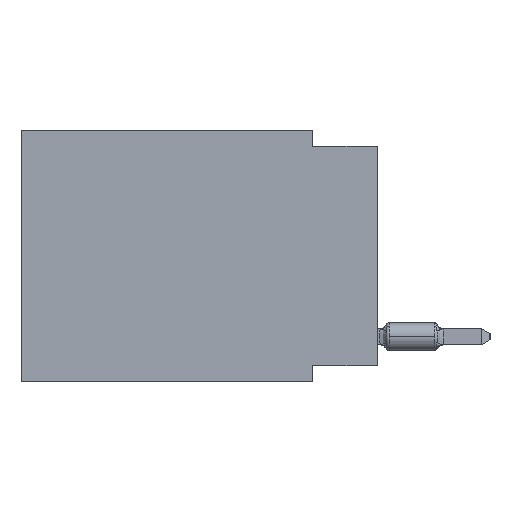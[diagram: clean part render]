
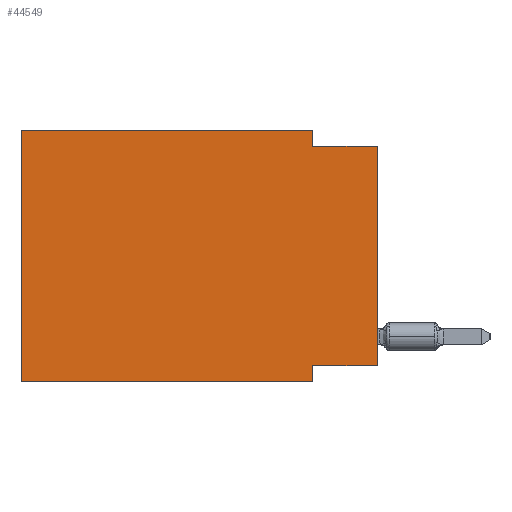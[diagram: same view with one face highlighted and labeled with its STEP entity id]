
A CAD part, left-side view. The second image highlights one B-rep face of the part: STEP entity #44549.
In plain terms, the highlighted planar face has unit normal (-1, 0, 0).
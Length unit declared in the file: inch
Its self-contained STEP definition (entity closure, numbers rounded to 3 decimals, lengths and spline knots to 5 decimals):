
#632 = CARTESIAN_POINT ( 'NONE',  ( 0., 0., -0.365 ) ) ;
#843 = ORIENTED_EDGE ( 'NONE', *, *, #45395, .F. ) ;
#1665 = VECTOR ( 'NONE', #24861, 39.37008 ) ;
#1793 = ORIENTED_EDGE ( 'NONE', *, *, #22220, .F. ) ;
#2018 = ORIENTED_EDGE ( 'NONE', *, *, #36033, .F. ) ;
#2411 = CARTESIAN_POINT ( 'NONE',  ( 0., 0.1, -0.39 ) ) ;
#2712 = LINE ( 'NONE', #18056, #1665 ) ;
#3088 = ORIENTED_EDGE ( 'NONE', *, *, #9856, .F. ) ;
#3418 = AXIS2_PLACEMENT_3D ( 'NONE', #48935, #29551, #9673 ) ;
#4784 = LINE ( 'NONE', #9063, #16529 ) ;
#4791 = EDGE_CURVE ( 'NONE', #34299, #46653, #4784, .T. ) ;
#5769 = CARTESIAN_POINT ( 'NONE',  ( 0., 0.1, -0.025 ) ) ;
#6405 = PLANE ( 'NONE',  #3418 ) ;
#6754 = VECTOR ( 'NONE', #19871, 39.37008 ) ;
#6849 = ORIENTED_EDGE ( 'NONE', *, *, #15875, .F. ) ;
#7074 = VECTOR ( 'NONE', #42676, 39.37008 ) ;
#7142 = CARTESIAN_POINT ( 'NONE',  ( 0., 0.1, -0.365 ) ) ;
#9063 = CARTESIAN_POINT ( 'NONE',  ( 0., 0., 0. ) ) ;
#9673 = DIRECTION ( 'NONE',  ( 0., 0., -1. ) ) ;
#9800 = DIRECTION ( 'NONE',  ( 0., -1., 0. ) ) ;
#9856 = EDGE_CURVE ( 'NONE', #13418, #49189, #2712, .T. ) ;
#10112 = ORIENTED_EDGE ( 'NONE', *, *, #24767, .F. ) ;
#11334 = VECTOR ( 'NONE', #27176, 39.37008 ) ;
#13418 = VERTEX_POINT ( 'NONE', #48258 ) ;
#14280 = DIRECTION ( 'NONE',  ( 0., 0., -1. ) ) ;
#14832 = CARTESIAN_POINT ( 'NONE',  ( 0., 0., -0.025 ) ) ;
#15875 = EDGE_CURVE ( 'NONE', #35598, #13418, #27934, .T. ) ;
#16285 = VECTOR ( 'NONE', #14280, 39.37008 ) ;
#16529 = VECTOR ( 'NONE', #39271, 39.37008 ) ;
#17598 = LINE ( 'NONE', #48317, #42395 ) ;
#18056 = CARTESIAN_POINT ( 'NONE',  ( 0., 0.55, 0. ) ) ;
#18533 = LINE ( 'NONE', #41215, #49306 ) ;
#19871 = DIRECTION ( 'NONE',  ( 0., 0., 1. ) ) ;
#19873 = ORIENTED_EDGE ( 'NONE', *, *, #4791, .T. ) ;
#20362 = VERTEX_POINT ( 'NONE', #5769 ) ;
#22220 = EDGE_CURVE ( 'NONE', #49189, #20362, #25886, .T. ) ;
#22844 = CARTESIAN_POINT ( 'NONE',  ( 0., 0.55, -0.39 ) ) ;
#23323 = CARTESIAN_POINT ( 'NONE',  ( 0., 0., -0.365 ) ) ;
#24149 = CARTESIAN_POINT ( 'NONE',  ( 0., 0.55, 0. ) ) ;
#24767 = EDGE_CURVE ( 'NONE', #20362, #46653, #17598, .T. ) ;
#24861 = DIRECTION ( 'NONE',  ( 0., -1., 0. ) ) ;
#25886 = LINE ( 'NONE', #41240, #16285 ) ;
#27076 = LINE ( 'NONE', #632, #7074 ) ;
#27176 = DIRECTION ( 'NONE',  ( 0., -1., 0. ) ) ;
#27934 = LINE ( 'NONE', #24149, #6754 ) ;
#29376 = CARTESIAN_POINT ( 'NONE',  ( 0., 0.1, 0. ) ) ;
#29551 = DIRECTION ( 'NONE',  ( 1., 0., 0. ) ) ;
#32112 = ORIENTED_EDGE ( 'NONE', *, *, #41341, .T. ) ;
#34299 = VERTEX_POINT ( 'NONE', #23323 ) ;
#35598 = VERTEX_POINT ( 'NONE', #22844 ) ;
#36033 = EDGE_CURVE ( 'NONE', #34299, #36347, #27076, .T. ) ;
#36347 = VERTEX_POINT ( 'NONE', #7142 ) ;
#39248 = LINE ( 'NONE', #47051, #11334 ) ;
#39271 = DIRECTION ( 'NONE',  ( 0., 0., 1. ) ) ;
#40220 = VERTEX_POINT ( 'NONE', #2411 ) ;
#41215 = CARTESIAN_POINT ( 'NONE',  ( 0., 0.1, -0.39 ) ) ;
#41240 = CARTESIAN_POINT ( 'NONE',  ( 0., 0.1, 0. ) ) ;
#41341 = EDGE_CURVE ( 'NONE', #35598, #40220, #39248, .T. ) ;
#42395 = VECTOR ( 'NONE', #9800, 39.37008 ) ;
#42676 = DIRECTION ( 'NONE',  ( 0., 1., 0. ) ) ;
#44549 = ADVANCED_FACE ( 'NONE', ( #47945 ), #6405, .F. ) ;
#45395 = EDGE_CURVE ( 'NONE', #36347, #40220, #18533, .T. ) ;
#46653 = VERTEX_POINT ( 'NONE', #14832 ) ;
#47051 = CARTESIAN_POINT ( 'NONE',  ( 0., 0.55, -0.39 ) ) ;
#47945 = FACE_OUTER_BOUND ( 'NONE', #49123, .T. ) ;
#48258 = CARTESIAN_POINT ( 'NONE',  ( 0., 0.55, 0. ) ) ;
#48317 = CARTESIAN_POINT ( 'NONE',  ( 0., 0., -0.025 ) ) ;
#48935 = CARTESIAN_POINT ( 'NONE',  ( 0., 0.55, 0. ) ) ;
#49002 = DIRECTION ( 'NONE',  ( 0., 0., -1. ) ) ;
#49123 = EDGE_LOOP ( 'NONE', ( #19873, #10112, #1793, #3088, #6849, #32112, #843, #2018 ) ) ;
#49189 = VERTEX_POINT ( 'NONE', #29376 ) ;
#49306 = VECTOR ( 'NONE', #49002, 39.37008 ) ;
